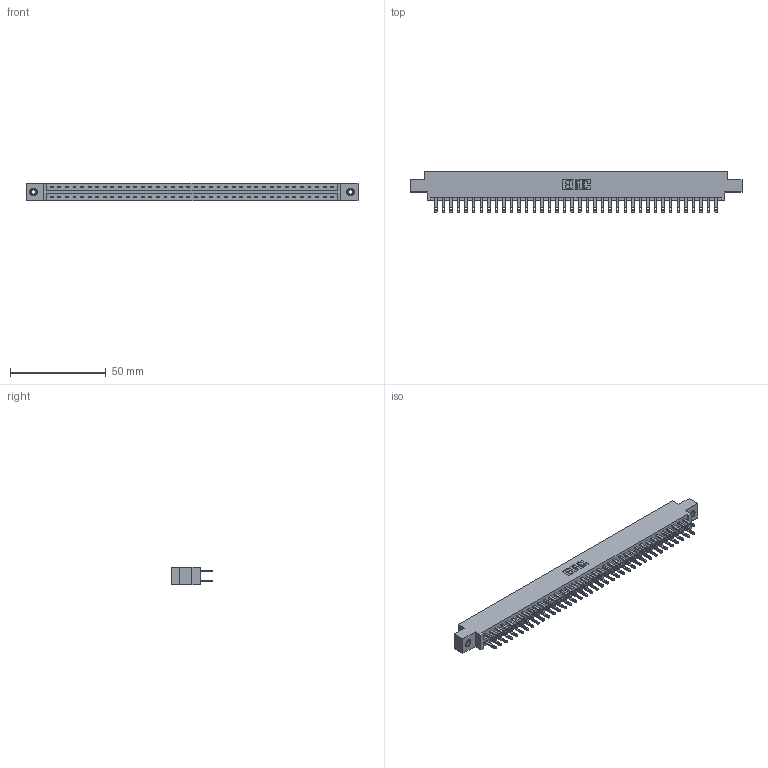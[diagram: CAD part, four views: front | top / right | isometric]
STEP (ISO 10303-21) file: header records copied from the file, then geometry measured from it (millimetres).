
FILE_DESCRIPTION (( 'STEP AP203' ), '1' );
FILE_NAME ('887-076-500-808.STEP', '2020-09-21T04:00:17', ( '' ), ( '' ), 'SwSTEP 2.0', 'SolidWorks 2020', '' );
FILE_SCHEMA (( 'CONFIG_CONTROL_DESIGN' ));
Length unit declared in the file: inch
Products named in the file (4): 345-250-001_345-250-003-102; 345-292-001_345-293-100; 887-076-500-808; 837 Part_0.170 Offset - 0.156 Dia-TI
Assembly tree (79 placements, depth 2):
  887-076-500-808
    837 Part_0.170 Offset - 0.156 Dia-TI
    345-292-001_345-293-100  x76
    345-250-001_345-250-003-102  x2
Bounding box: 173.58 x 21.85 x 9.4 mm (x, y, z)
Volume: 18348.6 mm3; surface area: 21679.3 mm2
Topology: 79 solids, 79 shells, 3978 faces, 12087 edges, 8050 vertices
Faces by surface type: plane 2538, cylinder 1424, cone 12, torus 4
Entity records: 31228 total; most frequent: CARTESIAN_POINT 5245, ORIENTED_EDGE 5174, DIRECTION 4501, EDGE_CURVE 2587, LINE 2435, VECTOR 2435, VERTEX_POINT 1720, AXIS2_PLACEMENT_3D 1033
